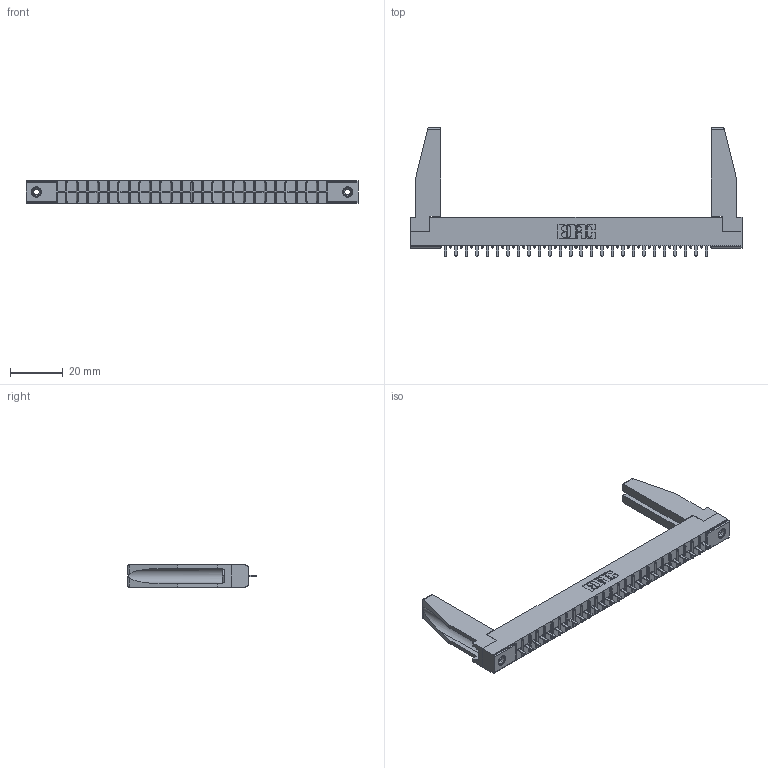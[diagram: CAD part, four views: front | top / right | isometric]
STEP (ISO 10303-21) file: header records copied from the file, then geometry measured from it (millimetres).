
FILE_DESCRIPTION (( 'STEP AP203' ), '1' );
FILE_NAME ('306-026-521-178.STEP', '2019-09-11T21:44:32', ( '' ), ( '' ), 'SwSTEP 2.0', 'SolidWorks 2016', '' );
FILE_SCHEMA (( 'CONFIG_CONTROL_DESIGN' ));
Length unit declared in the file: inch
Products named in the file (5): 306 Part_.156 Dia; 306-290-001_121; 345-250-001_345-250-001-102; 307-220-078; 306-026-521-178
Assembly tree (31 placements, depth 2):
  306-026-521-178
    306 Part_.156 Dia
    306-290-001_121  x26
    345-250-001_345-250-001-102  x2
    307-220-078  x2
Bounding box: 126.03 x 48.92 x 8.71 mm (x, y, z)
Volume: 12593.3 mm3; surface area: 16498.9 mm2
Topology: 31 solids, 31 shells, 2066 faces, 5768 edges, 3696 vertices
Faces by surface type: plane 1374, cylinder 572, sphere 104, cone 12, torus 4
Entity records: 28714 total; most frequent: CARTESIAN_POINT 4819, ORIENTED_EDGE 4734, DIRECTION 4705, EDGE_CURVE 2367, VECTOR 1845, LINE 1845, VERTEX_POINT 1502, AXIS2_PLACEMENT_3D 1430
